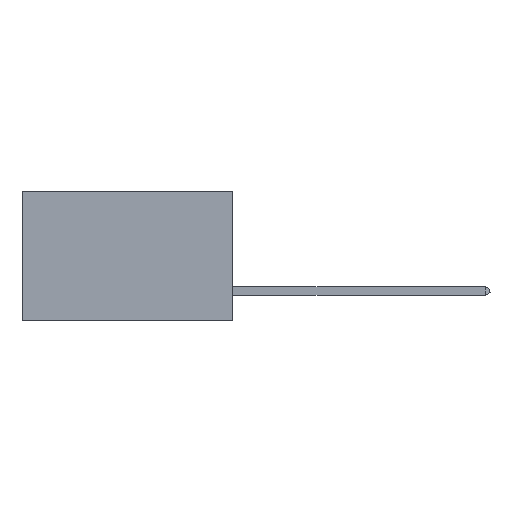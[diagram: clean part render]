
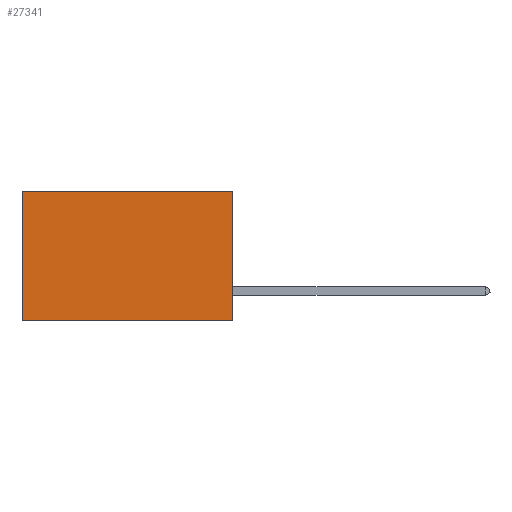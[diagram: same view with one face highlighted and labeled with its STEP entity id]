
A CAD part, left-side view. The second image highlights one B-rep face of the part: STEP entity #27341.
In plain terms, the highlighted planar face has unit normal (-1, 0, 0).
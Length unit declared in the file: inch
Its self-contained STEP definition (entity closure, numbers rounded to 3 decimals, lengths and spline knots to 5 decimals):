
#629 = LINE ( 'NONE', #10047, #21506 ) ;
#755 = VECTOR ( 'NONE', #9271, 39.37008 ) ;
#888 = CARTESIAN_POINT ( 'NONE',  ( 0.2875, 0.6, -0.37 ) ) ;
#1055 = CARTESIAN_POINT ( 'NONE',  ( 0.2875, 0., 0. ) ) ;
#1772 = LINE ( 'NONE', #14291, #34873 ) ;
#1864 = PLANE ( 'NONE',  #18104 ) ;
#4439 = DIRECTION ( 'NONE',  ( 1., 0., 0. ) ) ;
#5709 = LINE ( 'NONE', #15667, #22006 ) ;
#6025 = ORIENTED_EDGE ( 'NONE', *, *, #15318, .F. ) ;
#6500 = EDGE_CURVE ( 'NONE', #20827, #22290, #629, .T. ) ;
#7457 = DIRECTION ( 'NONE',  ( 0., 0., -1. ) ) ;
#8312 = ORIENTED_EDGE ( 'NONE', *, *, #6500, .F. ) ;
#9271 = DIRECTION ( 'NONE',  ( 0., 1., 0. ) ) ;
#9360 = EDGE_CURVE ( 'NONE', #30759, #10391, #5709, .T. ) ;
#9548 = CARTESIAN_POINT ( 'NONE',  ( 0.2875, 0., -0.37 ) ) ;
#10047 = CARTESIAN_POINT ( 'NONE',  ( 0.2875, 0., 0. ) ) ;
#10391 = VERTEX_POINT ( 'NONE', #888 ) ;
#13666 = EDGE_CURVE ( 'NONE', #20827, #30759, #1772, .T. ) ;
#14291 = CARTESIAN_POINT ( 'NONE',  ( 0.2875, 0., 0. ) ) ;
#15318 = EDGE_CURVE ( 'NONE', #22290, #10391, #32520, .T. ) ;
#15667 = CARTESIAN_POINT ( 'NONE',  ( 0.2875, 0.6, 0. ) ) ;
#18104 = AXIS2_PLACEMENT_3D ( 'NONE', #33577, #4439, #7457 ) ;
#18215 = DIRECTION ( 'NONE',  ( 0., 0., -1. ) ) ;
#20827 = VERTEX_POINT ( 'NONE', #1055 ) ;
#21506 = VECTOR ( 'NONE', #36153, 39.37008 ) ;
#22006 = VECTOR ( 'NONE', #18215, 39.37008 ) ;
#22290 = VERTEX_POINT ( 'NONE', #9548 ) ;
#23026 = DIRECTION ( 'NONE',  ( 0., 1., 0. ) ) ;
#23826 = ORIENTED_EDGE ( 'NONE', *, *, #9360, .T. ) ;
#26205 = EDGE_LOOP ( 'NONE', ( #23826, #6025, #8312, #31902 ) ) ;
#27341 = ADVANCED_FACE ( 'NONE', ( #37178 ), #1864, .F. ) ;
#29829 = CARTESIAN_POINT ( 'NONE',  ( 0.2875, 0., -0.37 ) ) ;
#29983 = CARTESIAN_POINT ( 'NONE',  ( 0.2875, 0.6, 0. ) ) ;
#30759 = VERTEX_POINT ( 'NONE', #29983 ) ;
#31902 = ORIENTED_EDGE ( 'NONE', *, *, #13666, .T. ) ;
#32520 = LINE ( 'NONE', #29829, #755 ) ;
#33577 = CARTESIAN_POINT ( 'NONE',  ( 0.2875, 0., 0. ) ) ;
#34873 = VECTOR ( 'NONE', #23026, 39.37008 ) ;
#36153 = DIRECTION ( 'NONE',  ( 0., 0., -1. ) ) ;
#37178 = FACE_OUTER_BOUND ( 'NONE', #26205, .T. ) ;
